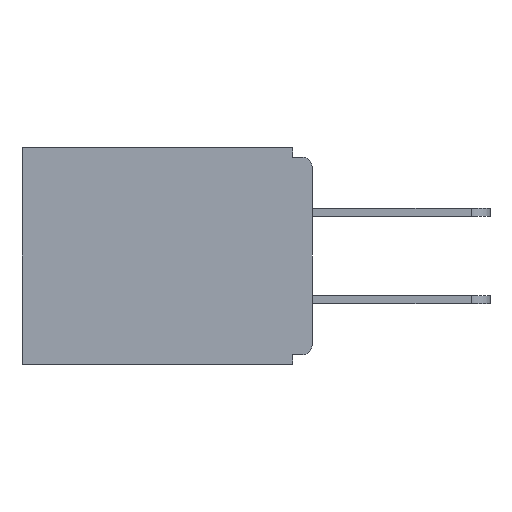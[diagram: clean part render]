
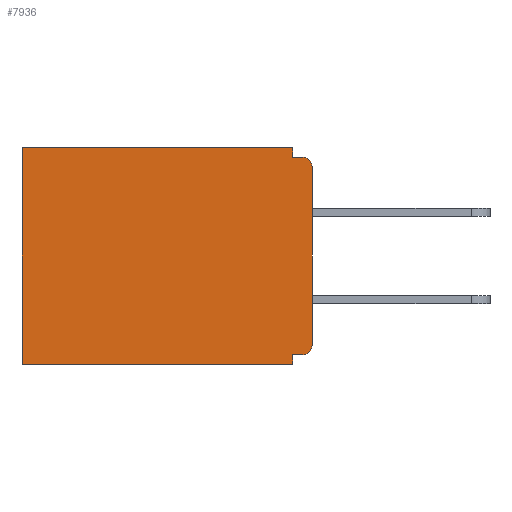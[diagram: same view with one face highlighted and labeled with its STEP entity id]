
A CAD part, left-side view. The second image highlights one B-rep face of the part: STEP entity #7936.
In plain terms, the highlighted planar face has unit normal (-1, 0, 0).
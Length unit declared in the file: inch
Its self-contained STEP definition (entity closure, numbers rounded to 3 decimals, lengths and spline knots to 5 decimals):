
#317 = EDGE_CURVE ( 'NONE', #2861, #2212, #4164, .T. ) ;
#476 = CARTESIAN_POINT ( 'NONE',  ( 0.298, 0.46, -0.343 ) ) ;
#574 = ORIENTED_EDGE ( 'NONE', *, *, #10502, .F. ) ;
#762 = PLANE ( 'NONE',  #3460 ) ;
#1299 = VERTEX_POINT ( 'NONE', #2663 ) ;
#1668 = DIRECTION ( 'NONE',  ( 0., 0., -1. ) ) ;
#1746 = VERTEX_POINT ( 'NONE', #9444 ) ;
#1751 = VECTOR ( 'NONE', #3721, 39.37008 ) ;
#2181 = DIRECTION ( 'NONE',  ( 0., 1., 0. ) ) ;
#2212 = VERTEX_POINT ( 'NONE', #6519 ) ;
#2410 = EDGE_CURVE ( 'NONE', #6497, #3444, #4673, .T. ) ;
#2473 = EDGE_CURVE ( 'NONE', #11557, #2932, #10382, .T. ) ;
#2546 = DIRECTION ( 'NONE',  ( -1., 0., 0. ) ) ;
#2663 = CARTESIAN_POINT ( 'NONE',  ( 0.298, 0.031, 0. ) ) ;
#2779 = DIRECTION ( 'NONE',  ( 0., 0., -1. ) ) ;
#2861 = VERTEX_POINT ( 'NONE', #6786 ) ;
#2932 = VERTEX_POINT ( 'NONE', #10129 ) ;
#3016 = ORIENTED_EDGE ( 'NONE', *, *, #5694, .F. ) ;
#3307 = AXIS2_PLACEMENT_3D ( 'NONE', #10573, #2546, #6158 ) ;
#3425 = CARTESIAN_POINT ( 'NONE',  ( 0.298, 0., 0. ) ) ;
#3444 = VERTEX_POINT ( 'NONE', #476 ) ;
#3460 = AXIS2_PLACEMENT_3D ( 'NONE', #3425, #6121, #1668 ) ;
#3639 = LINE ( 'NONE', #10796, #5875 ) ;
#3721 = DIRECTION ( 'NONE',  ( 0., -1., 0. ) ) ;
#3845 = EDGE_CURVE ( 'NONE', #1299, #2861, #3639, .T. ) ;
#4100 = VECTOR ( 'NONE', #7588, 39.37008 ) ;
#4133 = EDGE_CURVE ( 'NONE', #4838, #2932, #10211, .T. ) ;
#4164 = LINE ( 'NONE', #5493, #1751 ) ;
#4395 = VECTOR ( 'NONE', #7977, 39.37008 ) ;
#4624 = VECTOR ( 'NONE', #2181, 39.37008 ) ;
#4640 = CIRCLE ( 'NONE', #3307, 0.015 ) ;
#4673 = LINE ( 'NONE', #8484, #4100 ) ;
#4838 = VERTEX_POINT ( 'NONE', #6415 ) ;
#4916 = DIRECTION ( 'NONE',  ( 0., 0., -1. ) ) ;
#5071 = EDGE_CURVE ( 'NONE', #1299, #8172, #9436, .T. ) ;
#5391 = CARTESIAN_POINT ( 'NONE',  ( 0.298, 0.46, 0. ) ) ;
#5493 = CARTESIAN_POINT ( 'NONE',  ( 0.298, 0., -0.015 ) ) ;
#5694 = EDGE_CURVE ( 'NONE', #1746, #6497, #9132, .T. ) ;
#5875 = VECTOR ( 'NONE', #2779, 39.37008 ) ;
#6051 = CARTESIAN_POINT ( 'NONE',  ( 0.298, 0., 0. ) ) ;
#6094 = ORIENTED_EDGE ( 'NONE', *, *, #5071, .T. ) ;
#6121 = DIRECTION ( 'NONE',  ( 1., 0., 0. ) ) ;
#6158 = DIRECTION ( 'NONE',  ( 0., 0., -1. ) ) ;
#6245 = FACE_OUTER_BOUND ( 'NONE', #7969, .T. ) ;
#6353 = CARTESIAN_POINT ( 'NONE',  ( 0.298, 0.031, -0.343 ) ) ;
#6390 = ORIENTED_EDGE ( 'NONE', *, *, #3845, .F. ) ;
#6415 = CARTESIAN_POINT ( 'NONE',  ( 0.298, 0., -0.03 ) ) ;
#6497 = VERTEX_POINT ( 'NONE', #6353 ) ;
#6519 = CARTESIAN_POINT ( 'NONE',  ( 0.298, 0.015, -0.015 ) ) ;
#6786 = CARTESIAN_POINT ( 'NONE',  ( 0.298, 0.031, -0.015 ) ) ;
#6805 = EDGE_CURVE ( 'NONE', #4838, #2212, #4640, .T. ) ;
#6958 = ORIENTED_EDGE ( 'NONE', *, *, #4133, .F. ) ;
#7528 = LINE ( 'NONE', #11265, #4624 ) ;
#7578 = DIRECTION ( 'NONE',  ( 0., 0., -1. ) ) ;
#7587 = LINE ( 'NONE', #5391, #4395 ) ;
#7588 = DIRECTION ( 'NONE',  ( 0., 1., 0. ) ) ;
#7703 = CARTESIAN_POINT ( 'NONE',  ( 0.298, 0.015, -0.313 ) ) ;
#7820 = VECTOR ( 'NONE', #7578, 39.37008 ) ;
#7936 = ADVANCED_FACE ( 'NONE', ( #6245 ), #762, .F. ) ;
#7969 = EDGE_LOOP ( 'NONE', ( #10731, #10181, #6390, #6094, #10809, #10334, #3016, #574, #11191, #6958 ) ) ;
#7977 = DIRECTION ( 'NONE',  ( 0., 0., -1. ) ) ;
#8104 = EDGE_CURVE ( 'NONE', #8172, #3444, #7587, .T. ) ;
#8172 = VERTEX_POINT ( 'NONE', #9111 ) ;
#8484 = CARTESIAN_POINT ( 'NONE',  ( 0.298, 0., -0.343 ) ) ;
#8586 = VECTOR ( 'NONE', #11245, 39.37008 ) ;
#9031 = AXIS2_PLACEMENT_3D ( 'NONE', #7703, #10489, #11299 ) ;
#9111 = CARTESIAN_POINT ( 'NONE',  ( 0.298, 0.46, 0. ) ) ;
#9132 = LINE ( 'NONE', #11117, #10400 ) ;
#9436 = LINE ( 'NONE', #6051, #8586 ) ;
#9444 = CARTESIAN_POINT ( 'NONE',  ( 0.298, 0.031, -0.328 ) ) ;
#10129 = CARTESIAN_POINT ( 'NONE',  ( 0.298, 0., -0.313 ) ) ;
#10181 = ORIENTED_EDGE ( 'NONE', *, *, #317, .F. ) ;
#10211 = LINE ( 'NONE', #10363, #7820 ) ;
#10334 = ORIENTED_EDGE ( 'NONE', *, *, #2410, .F. ) ;
#10363 = CARTESIAN_POINT ( 'NONE',  ( 0.298, 0., 0. ) ) ;
#10382 = CIRCLE ( 'NONE', #9031, 0.015 ) ;
#10400 = VECTOR ( 'NONE', #4916, 39.37008 ) ;
#10476 = CARTESIAN_POINT ( 'NONE',  ( 0.298, 0.015, -0.328 ) ) ;
#10489 = DIRECTION ( 'NONE',  ( -1., 0., 0. ) ) ;
#10502 = EDGE_CURVE ( 'NONE', #11557, #1746, #7528, .T. ) ;
#10573 = CARTESIAN_POINT ( 'NONE',  ( 0.298, 0.015, -0.03 ) ) ;
#10731 = ORIENTED_EDGE ( 'NONE', *, *, #6805, .T. ) ;
#10796 = CARTESIAN_POINT ( 'NONE',  ( 0.298, 0.031, -0.343 ) ) ;
#10809 = ORIENTED_EDGE ( 'NONE', *, *, #8104, .T. ) ;
#11117 = CARTESIAN_POINT ( 'NONE',  ( 0.298, 0.031, -0.343 ) ) ;
#11191 = ORIENTED_EDGE ( 'NONE', *, *, #2473, .T. ) ;
#11245 = DIRECTION ( 'NONE',  ( 0., 1., 0. ) ) ;
#11265 = CARTESIAN_POINT ( 'NONE',  ( 0.298, 0., -0.328 ) ) ;
#11299 = DIRECTION ( 'NONE',  ( 0., 0., -1. ) ) ;
#11557 = VERTEX_POINT ( 'NONE', #10476 ) ;
